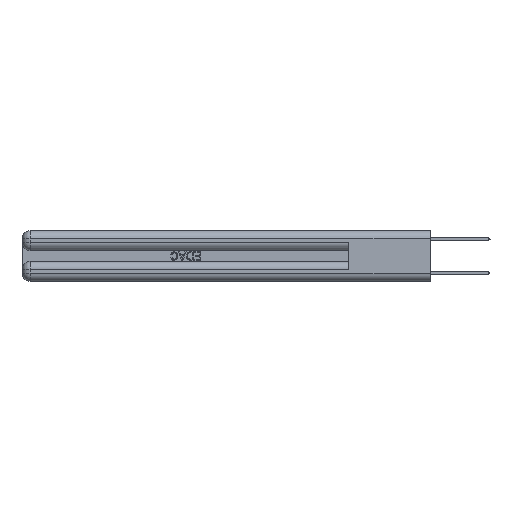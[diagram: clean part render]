
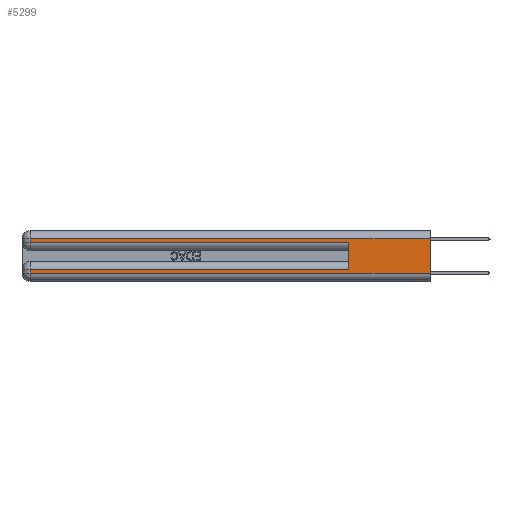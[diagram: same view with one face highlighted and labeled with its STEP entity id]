
A CAD part, left-side view. The second image highlights one B-rep face of the part: STEP entity #5299.
In plain terms, the highlighted planar face has unit normal (-1, 0, 0).
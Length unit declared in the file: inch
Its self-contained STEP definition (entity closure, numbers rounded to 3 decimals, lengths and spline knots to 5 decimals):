
#886 = VERTEX_POINT ( 'NONE', #7209 ) ;
#1021 = ORIENTED_EDGE ( 'NONE', *, *, #9262, .T. ) ;
#1330 = CARTESIAN_POINT ( 'NONE',  ( 0., 0., 0.37 ) ) ;
#1349 = VERTEX_POINT ( 'NONE', #4118 ) ;
#1373 = VERTEX_POINT ( 'NONE', #29940 ) ;
#1959 = VERTEX_POINT ( 'NONE', #23952 ) ;
#2362 = VERTEX_POINT ( 'NONE', #29581 ) ;
#2391 = CARTESIAN_POINT ( 'NONE',  ( 0., 0., 0.285 ) ) ;
#2567 = ORIENTED_EDGE ( 'NONE', *, *, #16409, .T. ) ;
#2888 = DIRECTION ( 'NONE',  ( 0., 0., -1. ) ) ;
#3840 = CARTESIAN_POINT ( 'NONE',  ( 0., 0.6, 0.145 ) ) ;
#4118 = CARTESIAN_POINT ( 'NONE',  ( 0., 2.94, 0.085 ) ) ;
#4255 = ORIENTED_EDGE ( 'NONE', *, *, #10753, .T. ) ;
#4540 = ORIENTED_EDGE ( 'NONE', *, *, #18330, .F. ) ;
#4707 = LINE ( 'NONE', #2391, #15594 ) ;
#5299 = ADVANCED_FACE ( 'NONE', ( #11793 ), #15557, .F. ) ;
#5501 = VECTOR ( 'NONE', #9624, 39.37008 ) ;
#6996 = CARTESIAN_POINT ( 'NONE',  ( 0., 0., 0.06 ) ) ;
#7209 = CARTESIAN_POINT ( 'NONE',  ( 0., 0.6, 0.085 ) ) ;
#7595 = ORIENTED_EDGE ( 'NONE', *, *, #17604, .T. ) ;
#8069 = AXIS2_PLACEMENT_3D ( 'NONE', #1330, #27281, #20177 ) ;
#8295 = VECTOR ( 'NONE', #2888, 39.37008 ) ;
#9262 = EDGE_CURVE ( 'NONE', #2362, #1959, #12885, .T. ) ;
#9580 = VECTOR ( 'NONE', #20932, 39.37008 ) ;
#9624 = DIRECTION ( 'NONE',  ( 0., -1., 0. ) ) ;
#10029 = EDGE_CURVE ( 'NONE', #886, #1349, #29159, .T. ) ;
#10753 = EDGE_CURVE ( 'NONE', #1373, #2362, #14645, .T. ) ;
#11039 = DIRECTION ( 'NONE',  ( 0., 0., -1. ) ) ;
#11377 = LINE ( 'NONE', #24848, #23265 ) ;
#11452 = VECTOR ( 'NONE', #26719, 39.37008 ) ;
#11793 = FACE_OUTER_BOUND ( 'NONE', #15867, .T. ) ;
#12885 = LINE ( 'NONE', #18800, #22638 ) ;
#13452 = ORIENTED_EDGE ( 'NONE', *, *, #25692, .F. ) ;
#14645 = LINE ( 'NONE', #20534, #9580 ) ;
#15001 = VERTEX_POINT ( 'NONE', #30028 ) ;
#15229 = EDGE_CURVE ( 'NONE', #1349, #15001, #11377, .T. ) ;
#15377 = VERTEX_POINT ( 'NONE', #27807 ) ;
#15557 = PLANE ( 'NONE',  #8069 ) ;
#15594 = VECTOR ( 'NONE', #18589, 39.37008 ) ;
#15867 = EDGE_LOOP ( 'NONE', ( #4540, #4255, #1021, #7595, #13452, #21566, #19708, #2567 ) ) ;
#16311 = DIRECTION ( 'NONE',  ( 0., 0., -1. ) ) ;
#16409 = EDGE_CURVE ( 'NONE', #15001, #15377, #25402, .T. ) ;
#17604 = EDGE_CURVE ( 'NONE', #1959, #18400, #4707, .T. ) ;
#18330 = EDGE_CURVE ( 'NONE', #1373, #15377, #29640, .T. ) ;
#18400 = VERTEX_POINT ( 'NONE', #28631 ) ;
#18589 = DIRECTION ( 'NONE',  ( 0., -1., 0. ) ) ;
#18800 = CARTESIAN_POINT ( 'NONE',  ( 0., 2.94, 0.37 ) ) ;
#19708 = ORIENTED_EDGE ( 'NONE', *, *, #15229, .T. ) ;
#20177 = DIRECTION ( 'NONE',  ( 0., 0., -1. ) ) ;
#20534 = CARTESIAN_POINT ( 'NONE',  ( 0., 0., 0.31 ) ) ;
#20932 = DIRECTION ( 'NONE',  ( 0., 1., 0. ) ) ;
#21566 = ORIENTED_EDGE ( 'NONE', *, *, #10029, .T. ) ;
#22638 = VECTOR ( 'NONE', #16311, 39.37008 ) ;
#22974 = VECTOR ( 'NONE', #28107, 39.37008 ) ;
#23265 = VECTOR ( 'NONE', #11039, 39.37008 ) ;
#23331 = LINE ( 'NONE', #3840, #11452 ) ;
#23952 = CARTESIAN_POINT ( 'NONE',  ( 0., 2.94, 0.285 ) ) ;
#24848 = CARTESIAN_POINT ( 'NONE',  ( 0., 2.94, 0.37 ) ) ;
#25402 = LINE ( 'NONE', #6996, #5501 ) ;
#25692 = EDGE_CURVE ( 'NONE', #886, #18400, #23331, .T. ) ;
#25764 = CARTESIAN_POINT ( 'NONE',  ( 0., 0., 0.085 ) ) ;
#25871 = CARTESIAN_POINT ( 'NONE',  ( 0., 0., 0.37 ) ) ;
#26719 = DIRECTION ( 'NONE',  ( 0., 0., 1. ) ) ;
#27281 = DIRECTION ( 'NONE',  ( 1., 0., 0. ) ) ;
#27807 = CARTESIAN_POINT ( 'NONE',  ( 0., 0., 0.06 ) ) ;
#28107 = DIRECTION ( 'NONE',  ( 0., 1., 0. ) ) ;
#28631 = CARTESIAN_POINT ( 'NONE',  ( 0., 0.6, 0.285 ) ) ;
#29159 = LINE ( 'NONE', #25764, #22974 ) ;
#29581 = CARTESIAN_POINT ( 'NONE',  ( 0., 2.94, 0.31 ) ) ;
#29640 = LINE ( 'NONE', #25871, #8295 ) ;
#29940 = CARTESIAN_POINT ( 'NONE',  ( 0., 0., 0.31 ) ) ;
#30028 = CARTESIAN_POINT ( 'NONE',  ( 0., 2.94, 0.06 ) ) ;
